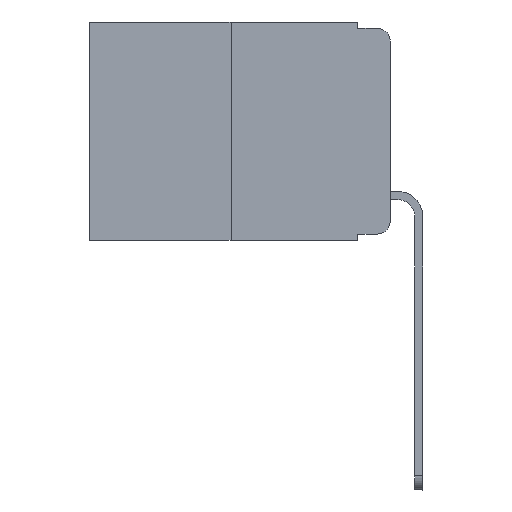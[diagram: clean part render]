
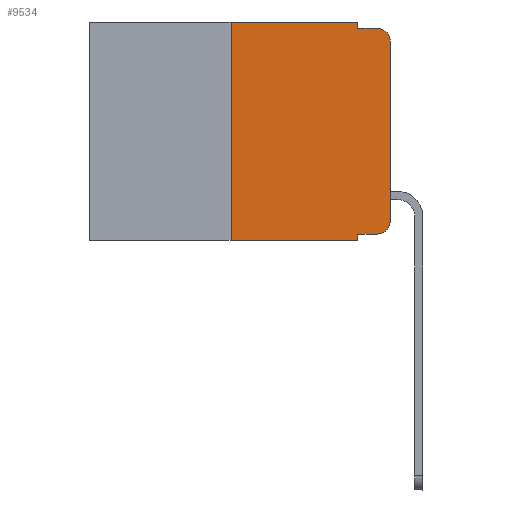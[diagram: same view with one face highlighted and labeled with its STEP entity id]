
A CAD part, left-side view. The second image highlights one B-rep face of the part: STEP entity #9534.
In plain terms, the highlighted planar face has unit normal (-1, 0, 0).
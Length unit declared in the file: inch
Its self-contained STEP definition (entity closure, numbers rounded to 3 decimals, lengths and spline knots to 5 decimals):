
#335 = VERTEX_POINT ( 'NONE', #8442 ) ;
#399 = DIRECTION ( 'NONE',  ( 0., 0., -1. ) ) ;
#479 = ORIENTED_EDGE ( 'NONE', *, *, #23823, .T. ) ;
#542 = VECTOR ( 'NONE', #20331, 39.37008 ) ;
#1172 = FACE_OUTER_BOUND ( 'NONE', #14108, .T. ) ;
#1542 = EDGE_CURVE ( 'NONE', #5237, #14377, #21081, .T. ) ;
#2737 = ORIENTED_EDGE ( 'NONE', *, *, #5661, .T. ) ;
#2818 = VECTOR ( 'NONE', #13620, 39.37008 ) ;
#3559 = LINE ( 'NONE', #21089, #15258 ) ;
#3770 = CIRCLE ( 'NONE', #20809, 0.02 ) ;
#4257 = LINE ( 'NONE', #15127, #15267 ) ;
#5237 = VERTEX_POINT ( 'NONE', #24205 ) ;
#5447 = DIRECTION ( 'NONE',  ( 0., -1., 0. ) ) ;
#5569 = DIRECTION ( 'NONE',  ( 0., 0., -1. ) ) ;
#5585 = VERTEX_POINT ( 'NONE', #6473 ) ;
#5629 = CARTESIAN_POINT ( 'NONE',  ( 0., 0., -0.03 ) ) ;
#5661 = EDGE_CURVE ( 'NONE', #19719, #14421, #3770, .T. ) ;
#5777 = CARTESIAN_POINT ( 'NONE',  ( 0., 0.02, -0.313 ) ) ;
#6351 = CARTESIAN_POINT ( 'NONE',  ( 0., 0.25, 0. ) ) ;
#6473 = CARTESIAN_POINT ( 'NONE',  ( 0., 0.051, -0.01 ) ) ;
#6602 = CARTESIAN_POINT ( 'NONE',  ( 0., 0.02, -0.03 ) ) ;
#6832 = VECTOR ( 'NONE', #399, 39.37008 ) ;
#7181 = EDGE_CURVE ( 'NONE', #8065, #9592, #4257, .T. ) ;
#7371 = LINE ( 'NONE', #15387, #2818 ) ;
#8065 = VERTEX_POINT ( 'NONE', #11845 ) ;
#8442 = CARTESIAN_POINT ( 'NONE',  ( 0., 0., -0.313 ) ) ;
#8497 = CARTESIAN_POINT ( 'NONE',  ( 0., 0.051, 0. ) ) ;
#8526 = DIRECTION ( 'NONE',  ( 0., 0., -1. ) ) ;
#9356 = EDGE_CURVE ( 'NONE', #14526, #5237, #24011, .T. ) ;
#9534 = ADVANCED_FACE ( 'NONE', ( #1172 ), #16533, .F. ) ;
#9592 = VERTEX_POINT ( 'NONE', #24781 ) ;
#11845 = CARTESIAN_POINT ( 'NONE',  ( 0., 0.051, -0.333 ) ) ;
#12248 = EDGE_CURVE ( 'NONE', #14526, #9592, #13795, .T. ) ;
#12849 = DIRECTION ( 'NONE',  ( 1., 0., 0. ) ) ;
#13279 = EDGE_CURVE ( 'NONE', #19780, #335, #24275, .T. ) ;
#13620 = DIRECTION ( 'NONE',  ( 0., -1., 0. ) ) ;
#13795 = LINE ( 'NONE', #17943, #15412 ) ;
#13830 = EDGE_CURVE ( 'NONE', #14377, #5585, #14258, .T. ) ;
#14066 = EDGE_CURVE ( 'NONE', #5585, #14421, #7371, .T. ) ;
#14108 = EDGE_LOOP ( 'NONE', ( #18445, #2737, #24725, #18319, #24351, #14494, #18949, #15109, #479, #17320 ) ) ;
#14258 = LINE ( 'NONE', #23519, #6832 ) ;
#14261 = VECTOR ( 'NONE', #22734, 39.37008 ) ;
#14377 = VERTEX_POINT ( 'NONE', #8497 ) ;
#14421 = VERTEX_POINT ( 'NONE', #22073 ) ;
#14494 = ORIENTED_EDGE ( 'NONE', *, *, #9356, .F. ) ;
#14517 = DIRECTION ( 'NONE',  ( -1., 0., 0. ) ) ;
#14526 = VERTEX_POINT ( 'NONE', #18846 ) ;
#15012 = CARTESIAN_POINT ( 'NONE',  ( 0., 0.473, 0. ) ) ;
#15109 = ORIENTED_EDGE ( 'NONE', *, *, #7181, .F. ) ;
#15127 = CARTESIAN_POINT ( 'NONE',  ( 0., 0.051, 0. ) ) ;
#15258 = VECTOR ( 'NONE', #5447, 39.37008 ) ;
#15267 = VECTOR ( 'NONE', #5569, 39.37008 ) ;
#15387 = CARTESIAN_POINT ( 'NONE',  ( 0., 0.051, -0.01 ) ) ;
#15412 = VECTOR ( 'NONE', #21521, 39.37008 ) ;
#15553 = CARTESIAN_POINT ( 'NONE',  ( 0., 0.02, -0.333 ) ) ;
#15760 = AXIS2_PLACEMENT_3D ( 'NONE', #5777, #17222, #21286 ) ;
#15996 = AXIS2_PLACEMENT_3D ( 'NONE', #15012, #12849, #24653 ) ;
#16533 = PLANE ( 'NONE',  #15996 ) ;
#17032 = CARTESIAN_POINT ( 'NONE',  ( 0., 0., 0. ) ) ;
#17222 = DIRECTION ( 'NONE',  ( -1., 0., 0. ) ) ;
#17320 = ORIENTED_EDGE ( 'NONE', *, *, #13279, .T. ) ;
#17714 = VECTOR ( 'NONE', #19421, 39.37008 ) ;
#17943 = CARTESIAN_POINT ( 'NONE',  ( 0., 0.473, -0.343 ) ) ;
#18319 = ORIENTED_EDGE ( 'NONE', *, *, #13830, .F. ) ;
#18445 = ORIENTED_EDGE ( 'NONE', *, *, #25043, .T. ) ;
#18846 = CARTESIAN_POINT ( 'NONE',  ( 0., 0.25, -0.343 ) ) ;
#18949 = ORIENTED_EDGE ( 'NONE', *, *, #12248, .T. ) ;
#19050 = LINE ( 'NONE', #17032, #14261 ) ;
#19421 = DIRECTION ( 'NONE',  ( 0., -1., 0. ) ) ;
#19719 = VERTEX_POINT ( 'NONE', #5629 ) ;
#19780 = VERTEX_POINT ( 'NONE', #15553 ) ;
#20331 = DIRECTION ( 'NONE',  ( 0., 0., 1. ) ) ;
#20809 = AXIS2_PLACEMENT_3D ( 'NONE', #6602, #14517, #8526 ) ;
#21081 = LINE ( 'NONE', #23472, #17714 ) ;
#21089 = CARTESIAN_POINT ( 'NONE',  ( 0., 0.051, -0.333 ) ) ;
#21286 = DIRECTION ( 'NONE',  ( 0., 0., -1. ) ) ;
#21521 = DIRECTION ( 'NONE',  ( 0., -1., 0. ) ) ;
#22073 = CARTESIAN_POINT ( 'NONE',  ( 0., 0.02, -0.01 ) ) ;
#22734 = DIRECTION ( 'NONE',  ( 0., 0., 1. ) ) ;
#23472 = CARTESIAN_POINT ( 'NONE',  ( 0., 0.473, 0. ) ) ;
#23519 = CARTESIAN_POINT ( 'NONE',  ( 0., 0.051, 0. ) ) ;
#23823 = EDGE_CURVE ( 'NONE', #8065, #19780, #3559, .T. ) ;
#24011 = LINE ( 'NONE', #6351, #542 ) ;
#24205 = CARTESIAN_POINT ( 'NONE',  ( 0., 0.25, 0. ) ) ;
#24275 = CIRCLE ( 'NONE', #15760, 0.02 ) ;
#24351 = ORIENTED_EDGE ( 'NONE', *, *, #1542, .F. ) ;
#24653 = DIRECTION ( 'NONE',  ( 0., 0., -1. ) ) ;
#24725 = ORIENTED_EDGE ( 'NONE', *, *, #14066, .F. ) ;
#24781 = CARTESIAN_POINT ( 'NONE',  ( 0., 0.051, -0.343 ) ) ;
#25043 = EDGE_CURVE ( 'NONE', #335, #19719, #19050, .T. ) ;
